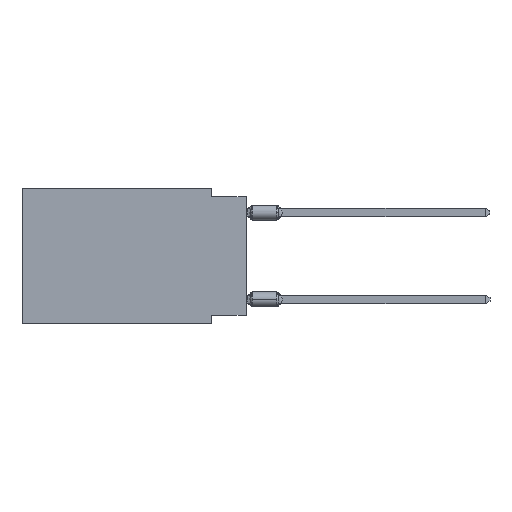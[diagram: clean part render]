
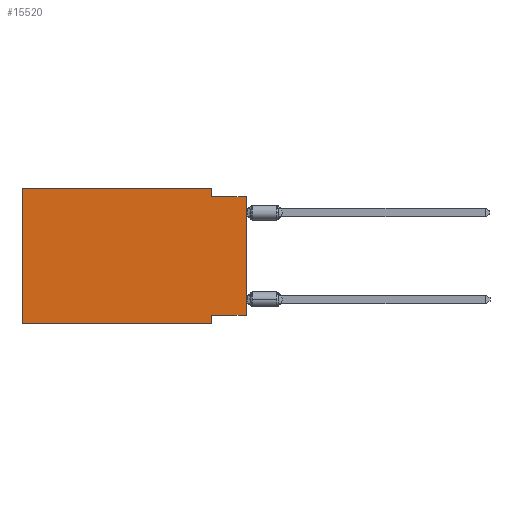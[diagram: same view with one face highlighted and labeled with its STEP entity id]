
A CAD part, left-side view. The second image highlights one B-rep face of the part: STEP entity #15520.
In plain terms, the highlighted planar face has unit normal (-1, 0, 0).
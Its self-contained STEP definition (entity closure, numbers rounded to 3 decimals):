
#54 = VECTOR ( 'NONE', #22126, 1000. ) ;
#1044 = LINE ( 'NONE', #24612, #24821 ) ;
#1344 = LINE ( 'NONE', #12100, #13762 ) ;
#1360 = CARTESIAN_POINT ( 'NONE',  ( 0., 2.54, -9.271 ) ) ;
#2254 = VECTOR ( 'NONE', #11728, 1000. ) ;
#2398 = VERTEX_POINT ( 'NONE', #26047 ) ;
#2499 = AXIS2_PLACEMENT_3D ( 'NONE', #10792, #19990, #15122 ) ;
#2930 = ORIENTED_EDGE ( 'NONE', *, *, #26427, .T. ) ;
#2952 = LINE ( 'NONE', #25057, #10460 ) ;
#3533 = VERTEX_POINT ( 'NONE', #17207 ) ;
#5156 = LINE ( 'NONE', #20355, #2254 ) ;
#8072 = CARTESIAN_POINT ( 'NONE',  ( 0., 2.54, -9.906 ) ) ;
#8385 = VERTEX_POINT ( 'NONE', #23523 ) ;
#10088 = VERTEX_POINT ( 'NONE', #13838 ) ;
#10445 = ORIENTED_EDGE ( 'NONE', *, *, #20421, .T. ) ;
#10460 = VECTOR ( 'NONE', #11685, 1000. ) ;
#10792 = CARTESIAN_POINT ( 'NONE',  ( 0., 16.383, 0. ) ) ;
#11100 = ORIENTED_EDGE ( 'NONE', *, *, #21229, .F. ) ;
#11158 = EDGE_LOOP ( 'NONE', ( #2930, #14180, #11100, #23716, #20139, #10445, #13110, #18418 ) ) ;
#11685 = DIRECTION ( 'NONE',  ( 0., 0., -1. ) ) ;
#11728 = DIRECTION ( 'NONE',  ( 0., 0., 1. ) ) ;
#12037 = VERTEX_POINT ( 'NONE', #24923 ) ;
#12100 = CARTESIAN_POINT ( 'NONE',  ( 0., 16.383, 0. ) ) ;
#12416 = EDGE_CURVE ( 'NONE', #18964, #3533, #1044, .T. ) ;
#13110 = ORIENTED_EDGE ( 'NONE', *, *, #25803, .F. ) ;
#13762 = VECTOR ( 'NONE', #27348, 1000. ) ;
#13838 = CARTESIAN_POINT ( 'NONE',  ( 0., 2.54, 0. ) ) ;
#13957 = VECTOR ( 'NONE', #16541, 1000. ) ;
#14114 = DIRECTION ( 'NONE',  ( 0., -1., 0. ) ) ;
#14180 = ORIENTED_EDGE ( 'NONE', *, *, #12416, .F. ) ;
#14658 = LINE ( 'NONE', #16550, #28114 ) ;
#15122 = DIRECTION ( 'NONE',  ( 0., 0., -1. ) ) ;
#15520 = ADVANCED_FACE ( 'NONE', ( #26459 ), #28321, .F. ) ;
#15532 = LINE ( 'NONE', #23708, #54 ) ;
#15811 = EDGE_CURVE ( 'NONE', #2398, #27015, #16968, .T. ) ;
#16501 = VECTOR ( 'NONE', #24247, 1000. ) ;
#16541 = DIRECTION ( 'NONE',  ( 0., 1., 0. ) ) ;
#16550 = CARTESIAN_POINT ( 'NONE',  ( 0., 2.54, 0. ) ) ;
#16968 = LINE ( 'NONE', #21530, #13957 ) ;
#17207 = CARTESIAN_POINT ( 'NONE',  ( 0., 0., -0.635 ) ) ;
#17330 = CARTESIAN_POINT ( 'NONE',  ( 0., 2.54, -0.635 ) ) ;
#18418 = ORIENTED_EDGE ( 'NONE', *, *, #15811, .F. ) ;
#18517 = EDGE_CURVE ( 'NONE', #8385, #12037, #1344, .T. ) ;
#18964 = VERTEX_POINT ( 'NONE', #17330 ) ;
#19990 = DIRECTION ( 'NONE',  ( 1., 0., 0. ) ) ;
#20139 = ORIENTED_EDGE ( 'NONE', *, *, #18517, .F. ) ;
#20355 = CARTESIAN_POINT ( 'NONE',  ( 0., 0., 0. ) ) ;
#20421 = EDGE_CURVE ( 'NONE', #8385, #21272, #26972, .T. ) ;
#21229 = EDGE_CURVE ( 'NONE', #10088, #18964, #14658, .T. ) ;
#21272 = VERTEX_POINT ( 'NONE', #8072 ) ;
#21530 = CARTESIAN_POINT ( 'NONE',  ( 0., 0., -9.271 ) ) ;
#22126 = DIRECTION ( 'NONE',  ( 0., -1., 0. ) ) ;
#22232 = CARTESIAN_POINT ( 'NONE',  ( 0., 16.383, -9.906 ) ) ;
#22682 = EDGE_CURVE ( 'NONE', #12037, #10088, #15532, .T. ) ;
#23140 = DIRECTION ( 'NONE',  ( 0., 0., -1. ) ) ;
#23523 = CARTESIAN_POINT ( 'NONE',  ( 0., 16.383, -9.906 ) ) ;
#23708 = CARTESIAN_POINT ( 'NONE',  ( 0., 16.383, 0. ) ) ;
#23716 = ORIENTED_EDGE ( 'NONE', *, *, #22682, .F. ) ;
#24247 = DIRECTION ( 'NONE',  ( 0., -1., 0. ) ) ;
#24612 = CARTESIAN_POINT ( 'NONE',  ( 0., 0., -0.635 ) ) ;
#24821 = VECTOR ( 'NONE', #14114, 1000. ) ;
#24923 = CARTESIAN_POINT ( 'NONE',  ( 0., 16.383, 0. ) ) ;
#25057 = CARTESIAN_POINT ( 'NONE',  ( 0., 2.54, -9.906 ) ) ;
#25803 = EDGE_CURVE ( 'NONE', #27015, #21272, #2952, .T. ) ;
#26047 = CARTESIAN_POINT ( 'NONE',  ( 0., 0., -9.271 ) ) ;
#26427 = EDGE_CURVE ( 'NONE', #2398, #3533, #5156, .T. ) ;
#26459 = FACE_OUTER_BOUND ( 'NONE', #11158, .T. ) ;
#26972 = LINE ( 'NONE', #22232, #16501 ) ;
#27015 = VERTEX_POINT ( 'NONE', #1360 ) ;
#27348 = DIRECTION ( 'NONE',  ( 0., 0., 1. ) ) ;
#28114 = VECTOR ( 'NONE', #23140, 1000. ) ;
#28321 = PLANE ( 'NONE',  #2499 ) ;
